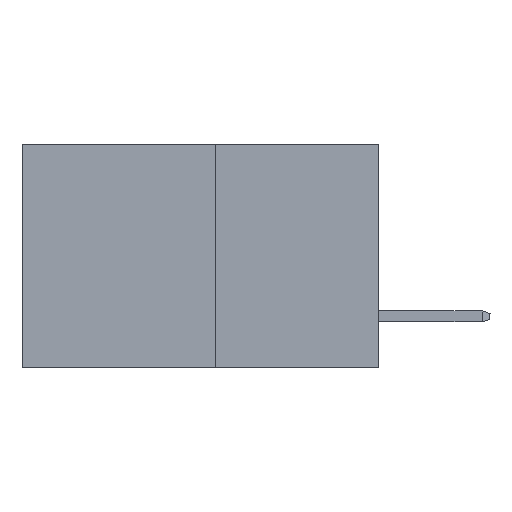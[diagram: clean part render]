
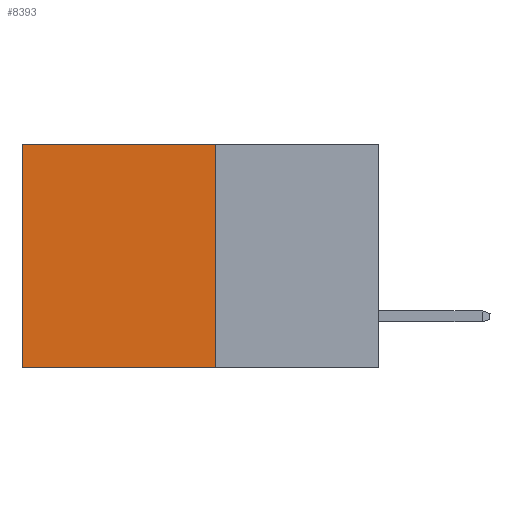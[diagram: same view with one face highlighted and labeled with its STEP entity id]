
A CAD part, left-side view. The second image highlights one B-rep face of the part: STEP entity #8393.
In plain terms, the highlighted planar face has unit normal (-1, 0, 0).
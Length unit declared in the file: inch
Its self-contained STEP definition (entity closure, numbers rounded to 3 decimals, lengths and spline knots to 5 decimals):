
#90 = EDGE_CURVE ( 'NONE', #13641, #8828, #1819, .T. ) ;
#219 = CARTESIAN_POINT ( 'NONE',  ( 0.277, 0.27, -0.37 ) ) ;
#466 = ORIENTED_EDGE ( 'NONE', *, *, #12145, .F. ) ;
#480 = EDGE_CURVE ( 'NONE', #13641, #13919, #12897, .T. ) ;
#798 = EDGE_CURVE ( 'NONE', #13919, #11511, #8617, .T. ) ;
#1625 = PLANE ( 'NONE',  #7767 ) ;
#1819 = LINE ( 'NONE', #219, #2265 ) ;
#1850 = CARTESIAN_POINT ( 'NONE',  ( 0.277, 0.59, -0.37 ) ) ;
#2265 = VECTOR ( 'NONE', #7391, 39.37008 ) ;
#2919 = ORIENTED_EDGE ( 'NONE', *, *, #798, .T. ) ;
#3010 = DIRECTION ( 'NONE',  ( 0., 0., -1. ) ) ;
#4074 = CARTESIAN_POINT ( 'NONE',  ( 0.277, 0.59, -0.37 ) ) ;
#4284 = VECTOR ( 'NONE', #6933, 39.37008 ) ;
#5234 = CARTESIAN_POINT ( 'NONE',  ( 0.277, 0.27, -0.37 ) ) ;
#5964 = ORIENTED_EDGE ( 'NONE', *, *, #480, .T. ) ;
#6833 = EDGE_LOOP ( 'NONE', ( #2919, #466, #13117, #5964 ) ) ;
#6933 = DIRECTION ( 'NONE',  ( 0., 1., 0. ) ) ;
#6991 = CARTESIAN_POINT ( 'NONE',  ( 0.277, 0.27, 0. ) ) ;
#7391 = DIRECTION ( 'NONE',  ( 0., 0., -1. ) ) ;
#7767 = AXIS2_PLACEMENT_3D ( 'NONE', #5234, #9689, #3010 ) ;
#8393 = ADVANCED_FACE ( 'NONE', ( #11103 ), #1625, .F. ) ;
#8617 = LINE ( 'NONE', #1850, #13819 ) ;
#8828 = VERTEX_POINT ( 'NONE', #14169 ) ;
#9004 = VECTOR ( 'NONE', #10173, 39.37008 ) ;
#9689 = DIRECTION ( 'NONE',  ( 1., 0., 0. ) ) ;
#9743 = CARTESIAN_POINT ( 'NONE',  ( 0.277, 0.27, 0. ) ) ;
#10127 = CARTESIAN_POINT ( 'NONE',  ( 0.277, 0.27, -0.37 ) ) ;
#10173 = DIRECTION ( 'NONE',  ( 0., 1., 0. ) ) ;
#11062 = CARTESIAN_POINT ( 'NONE',  ( 0.277, 0.59, 0. ) ) ;
#11103 = FACE_OUTER_BOUND ( 'NONE', #6833, .T. ) ;
#11127 = DIRECTION ( 'NONE',  ( 0., 0., -1. ) ) ;
#11511 = VERTEX_POINT ( 'NONE', #4074 ) ;
#12145 = EDGE_CURVE ( 'NONE', #8828, #11511, #13202, .T. ) ;
#12897 = LINE ( 'NONE', #6991, #4284 ) ;
#13117 = ORIENTED_EDGE ( 'NONE', *, *, #90, .F. ) ;
#13202 = LINE ( 'NONE', #10127, #9004 ) ;
#13641 = VERTEX_POINT ( 'NONE', #9743 ) ;
#13819 = VECTOR ( 'NONE', #11127, 39.37008 ) ;
#13919 = VERTEX_POINT ( 'NONE', #11062 ) ;
#14169 = CARTESIAN_POINT ( 'NONE',  ( 0.277, 0.27, -0.37 ) ) ;
